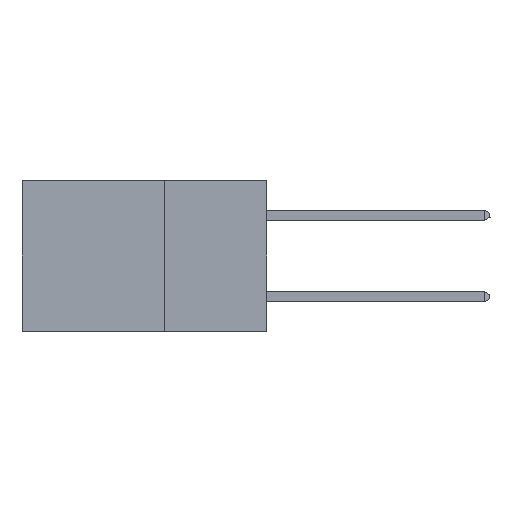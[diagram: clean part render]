
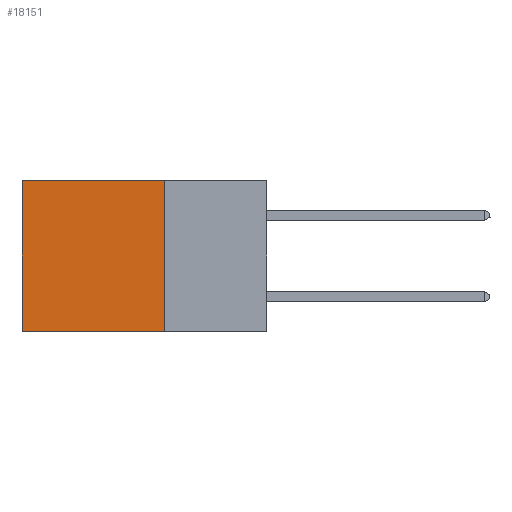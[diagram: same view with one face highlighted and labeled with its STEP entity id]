
A CAD part, left-side view. The second image highlights one B-rep face of the part: STEP entity #18151.
In plain terms, the highlighted planar face has unit normal (-1, 0, 0).
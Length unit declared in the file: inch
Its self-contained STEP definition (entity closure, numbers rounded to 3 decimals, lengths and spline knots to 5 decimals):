
#3044 = DIRECTION ( 'NONE',  ( 0., 0., -1. ) ) ;
#3249 = VERTEX_POINT ( 'NONE', #23700 ) ;
#3832 = VERTEX_POINT ( 'NONE', #26284 ) ;
#7555 = ORIENTED_EDGE ( 'NONE', *, *, #22262, .F. ) ;
#7937 = ORIENTED_EDGE ( 'NONE', *, *, #9162, .F. ) ;
#9162 = EDGE_CURVE ( 'NONE', #3249, #41707, #36696, .T. ) ;
#10314 = VECTOR ( 'NONE', #21798, 39.37008 ) ;
#10784 = ORIENTED_EDGE ( 'NONE', *, *, #20334, .T. ) ;
#11060 = CARTESIAN_POINT ( 'NONE',  ( 0.2875, 0.25, 0. ) ) ;
#11730 = LINE ( 'NONE', #15645, #27942 ) ;
#12377 = DIRECTION ( 'NONE',  ( 0., 1., 0. ) ) ;
#13553 = AXIS2_PLACEMENT_3D ( 'NONE', #11060, #13909, #18054 ) ;
#13909 = DIRECTION ( 'NONE',  ( 1., 0., 0. ) ) ;
#15015 = LINE ( 'NONE', #34912, #10314 ) ;
#15645 = CARTESIAN_POINT ( 'NONE',  ( 0.2875, 0.25, 0. ) ) ;
#15755 = LINE ( 'NONE', #32813, #21361 ) ;
#17833 = PLANE ( 'NONE',  #13553 ) ;
#18054 = DIRECTION ( 'NONE',  ( 0., 0., -1. ) ) ;
#18151 = ADVANCED_FACE ( 'NONE', ( #40544 ), #17833, .F. ) ;
#19390 = CARTESIAN_POINT ( 'NONE',  ( 0.2875, 0.6, 0. ) ) ;
#19626 = CARTESIAN_POINT ( 'NONE',  ( 0.2875, 0.25, -0.37 ) ) ;
#20334 = EDGE_CURVE ( 'NONE', #39110, #3832, #15755, .T. ) ;
#21361 = VECTOR ( 'NONE', #29102, 39.37008 ) ;
#21798 = DIRECTION ( 'NONE',  ( 0., 1., 0. ) ) ;
#22262 = EDGE_CURVE ( 'NONE', #41707, #3832, #15015, .T. ) ;
#23700 = CARTESIAN_POINT ( 'NONE',  ( 0.2875, 0.25, 0. ) ) ;
#26284 = CARTESIAN_POINT ( 'NONE',  ( 0.2875, 0.6, -0.37 ) ) ;
#27942 = VECTOR ( 'NONE', #12377, 39.37008 ) ;
#29102 = DIRECTION ( 'NONE',  ( 0., 0., -1. ) ) ;
#32033 = ORIENTED_EDGE ( 'NONE', *, *, #33659, .T. ) ;
#32515 = VECTOR ( 'NONE', #3044, 39.37008 ) ;
#32813 = CARTESIAN_POINT ( 'NONE',  ( 0.2875, 0.6, 0. ) ) ;
#33659 = EDGE_CURVE ( 'NONE', #3249, #39110, #11730, .T. ) ;
#34912 = CARTESIAN_POINT ( 'NONE',  ( 0.2875, 0.25, -0.37 ) ) ;
#36478 = CARTESIAN_POINT ( 'NONE',  ( 0.2875, 0.25, 0. ) ) ;
#36696 = LINE ( 'NONE', #36478, #32515 ) ;
#39110 = VERTEX_POINT ( 'NONE', #19390 ) ;
#39288 = EDGE_LOOP ( 'NONE', ( #10784, #7555, #7937, #32033 ) ) ;
#40544 = FACE_OUTER_BOUND ( 'NONE', #39288, .T. ) ;
#41707 = VERTEX_POINT ( 'NONE', #19626 ) ;
